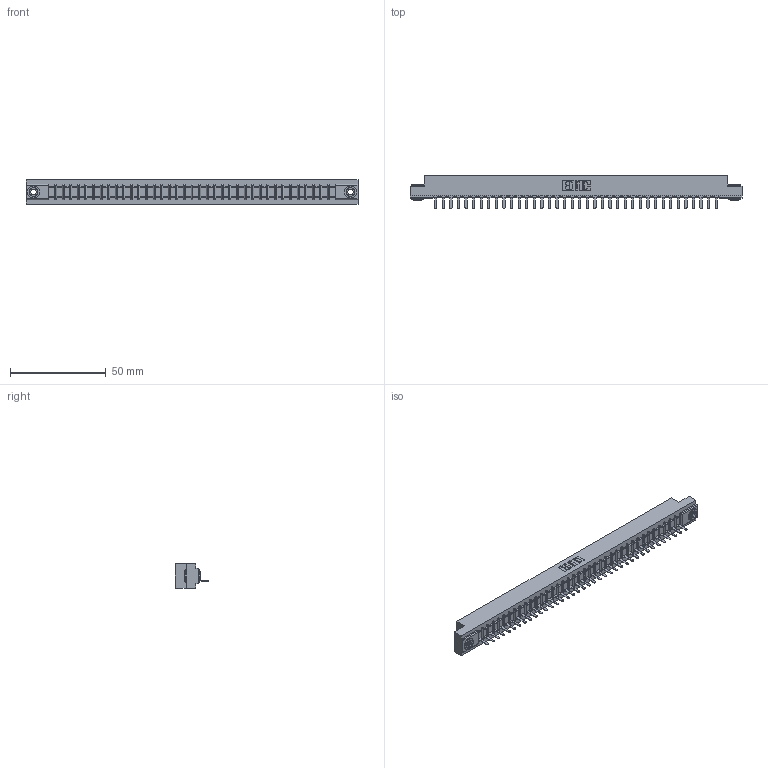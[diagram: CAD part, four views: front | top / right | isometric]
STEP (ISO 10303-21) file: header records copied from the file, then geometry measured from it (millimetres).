
FILE_DESCRIPTION (( 'STEP AP203' ), '1' );
FILE_NAME ('307-038-521-103.STEP', '2019-09-05T08:58:06', ( '' ), ( '' ), 'SwSTEP 2.0', 'SolidWorks 2016', '' );
FILE_SCHEMA (( 'CONFIG_CONTROL_DESIGN' ));
Length unit declared in the file: inch
Products named in the file (4): 307-290-002_521; 345-250-002_345-250-002-102; 307-038-521-103; 307 Part_.156 Dia Mounting Holes
Assembly tree (41 placements, depth 2):
  307-038-521-103
    307 Part_.156 Dia Mounting Holes
    307-290-002_521  x38
    345-250-002_345-250-002-102  x2
Bounding box: 173.58 x 17.42 x 12.7 mm (x, y, z)
Volume: 18549.3 mm3; surface area: 23491.1 mm2
Topology: 41 solids, 41 shells, 3021 faces, 9251 edges, 6058 vertices
Faces by surface type: plane 1804, cylinder 1131, sphere 78, cone 8
Entity records: 34853 total; most frequent: CARTESIAN_POINT 5857, ORIENTED_EDGE 5838, DIRECTION 5707, EDGE_CURVE 2919, VECTOR 2227, LINE 2227, VERTEX_POINT 1890, AXIS2_PLACEMENT_3D 1740
